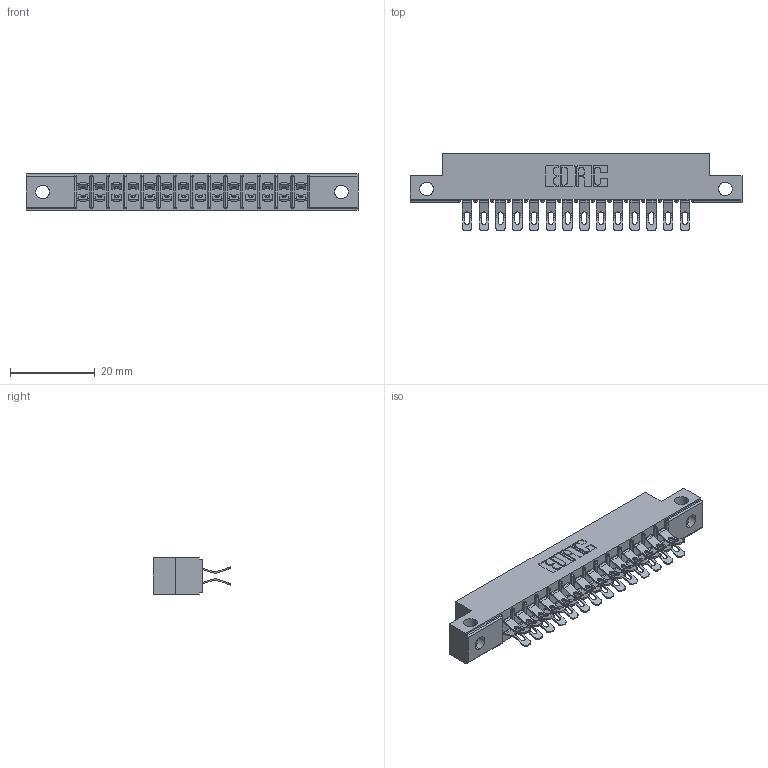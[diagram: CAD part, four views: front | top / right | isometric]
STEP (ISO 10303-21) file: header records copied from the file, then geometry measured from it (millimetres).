
FILE_DESCRIPTION (( 'STEP AP203' ), '1' );
FILE_NAME ('305-028-555-512.STEP', '2020-09-19T21:15:24', ( '' ), ( '' ), 'SwSTEP 2.0', 'SolidWorks 2020', '' );
FILE_SCHEMA (( 'CONFIG_CONTROL_DESIGN' ));
Length unit declared in the file: inch
Products named in the file (3): 305 Part_.128 Dia; 305-290-001_555; 305-028-555-512
Assembly tree (29 placements, depth 2):
  305-028-555-512
    305 Part_.128 Dia
    305-290-001_555  x28
Bounding box: 78.49 x 18.41 x 8.71 mm (x, y, z)
Volume: 4682 mm3; surface area: 9290.9 mm2
Topology: 29 solids, 29 shells, 1976 faces, 5882 edges, 3840 vertices
Faces by surface type: plane 964, cylinder 956, sphere 56
Entity records: 19597 total; most frequent: CARTESIAN_POINT 3310, ORIENTED_EDGE 3228, DIRECTION 3158, EDGE_CURVE 1614, LINE 1238, VECTOR 1238, VERTEX_POINT 1032, AXIS2_PLACEMENT_3D 960
